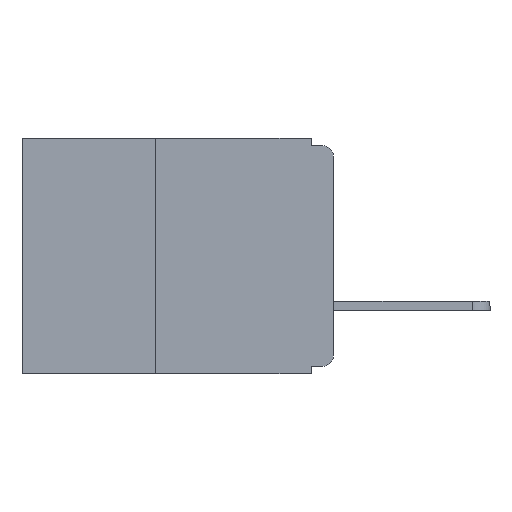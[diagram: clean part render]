
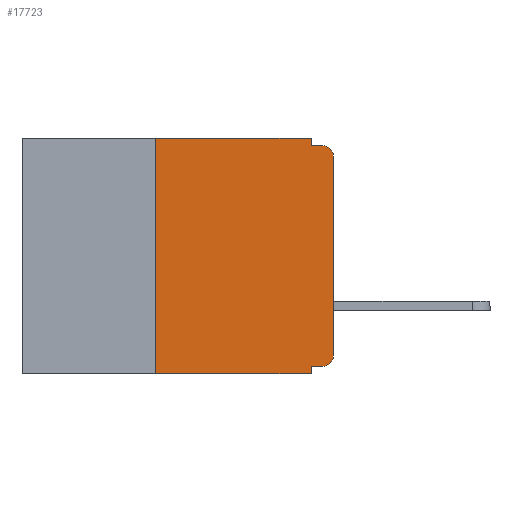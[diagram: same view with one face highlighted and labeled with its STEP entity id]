
A CAD part, left-side view. The second image highlights one B-rep face of the part: STEP entity #17723.
In plain terms, the highlighted planar face has unit normal (-1, 0, 0).
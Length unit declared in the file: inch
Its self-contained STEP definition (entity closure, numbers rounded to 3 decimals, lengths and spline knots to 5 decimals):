
#529 = AXIS2_PLACEMENT_3D ( 'NONE', #19629, #15218, #2746 ) ;
#1301 = EDGE_CURVE ( 'NONE', #6737, #12225, #20094, .T. ) ;
#1304 = AXIS2_PLACEMENT_3D ( 'NONE', #9690, #3925, #2881 ) ;
#1954 = VERTEX_POINT ( 'NONE', #9697 ) ;
#2313 = EDGE_CURVE ( 'NONE', #10436, #1954, #17542, .T. ) ;
#2382 = EDGE_CURVE ( 'NONE', #9512, #3164, #15989, .T. ) ;
#2688 = EDGE_CURVE ( 'NONE', #3176, #16818, #7140, .T. ) ;
#2746 = DIRECTION ( 'NONE',  ( 0., 0., -1. ) ) ;
#2881 = DIRECTION ( 'NONE',  ( 0., 0., -1. ) ) ;
#3124 = VECTOR ( 'NONE', #14455, 39.37008 ) ;
#3146 = LINE ( 'NONE', #15169, #3124 ) ;
#3164 = VERTEX_POINT ( 'NONE', #4464 ) ;
#3176 = VERTEX_POINT ( 'NONE', #18216 ) ;
#3925 = DIRECTION ( 'NONE',  ( -1., 0., 0. ) ) ;
#3968 = EDGE_LOOP ( 'NONE', ( #12111, #12404, #12671, #12971, #13162, #13450, #13623, #13916, #14060, #14146 ) ) ;
#4005 = DIRECTION ( 'NONE',  ( 0., -1., 0. ) ) ;
#4006 = VECTOR ( 'NONE', #19740, 39.37008 ) ;
#4296 = CARTESIAN_POINT ( 'NONE',  ( 0., 0., -0.01 ) ) ;
#4464 = CARTESIAN_POINT ( 'NONE',  ( 0., 0., -0.305 ) ) ;
#4554 = LINE ( 'NONE', #20011, #4006 ) ;
#4828 = CARTESIAN_POINT ( 'NONE',  ( 0., 0., 0. ) ) ;
#5099 = LINE ( 'NONE', #7003, #6762 ) ;
#5101 = DIRECTION ( 'NONE',  ( 0., 0., 1. ) ) ;
#5214 = CARTESIAN_POINT ( 'NONE',  ( 0., 0.031, 0. ) ) ;
#6737 = VERTEX_POINT ( 'NONE', #10512 ) ;
#6762 = VECTOR ( 'NONE', #7384, 39.37008 ) ;
#6795 = VERTEX_POINT ( 'NONE', #8122 ) ;
#7003 = CARTESIAN_POINT ( 'NONE',  ( 0., 0.031, 0. ) ) ;
#7140 = CIRCLE ( 'NONE', #1304, 0.015 ) ;
#7384 = DIRECTION ( 'NONE',  ( 0., 0., -1. ) ) ;
#7558 = DIRECTION ( 'NONE',  ( 0., 0., 1. ) ) ;
#8009 = VERTEX_POINT ( 'NONE', #5214 ) ;
#8122 = CARTESIAN_POINT ( 'NONE',  ( 0., 0.031, -0.01 ) ) ;
#9164 = EDGE_CURVE ( 'NONE', #6795, #16818, #11455, .T. ) ;
#9512 = VERTEX_POINT ( 'NONE', #19906 ) ;
#9690 = CARTESIAN_POINT ( 'NONE',  ( 0., 0.015, -0.025 ) ) ;
#9697 = CARTESIAN_POINT ( 'NONE',  ( 0., 0.25, 0. ) ) ;
#10065 = CARTESIAN_POINT ( 'NONE',  ( 0., 0.031, -0.33 ) ) ;
#10436 = VERTEX_POINT ( 'NONE', #17234 ) ;
#10447 = LINE ( 'NONE', #19452, #10653 ) ;
#10512 = CARTESIAN_POINT ( 'NONE',  ( 0., 0.031, -0.32 ) ) ;
#10653 = VECTOR ( 'NONE', #19446, 39.37008 ) ;
#11354 = VECTOR ( 'NONE', #4005, 39.37008 ) ;
#11455 = LINE ( 'NONE', #4296, #11354 ) ;
#12111 = ORIENTED_EDGE ( 'NONE', *, *, #13014, .T. ) ;
#12225 = VERTEX_POINT ( 'NONE', #10065 ) ;
#12404 = ORIENTED_EDGE ( 'NONE', *, *, #2688, .T. ) ;
#12595 = CARTESIAN_POINT ( 'NONE',  ( 0., 0.25, -0.33 ) ) ;
#12671 = ORIENTED_EDGE ( 'NONE', *, *, #9164, .F. ) ;
#12971 = ORIENTED_EDGE ( 'NONE', *, *, #20355, .F. ) ;
#13014 = EDGE_CURVE ( 'NONE', #3164, #3176, #13865, .T. ) ;
#13162 = ORIENTED_EDGE ( 'NONE', *, *, #18551, .F. ) ;
#13450 = ORIENTED_EDGE ( 'NONE', *, *, #2313, .F. ) ;
#13623 = ORIENTED_EDGE ( 'NONE', *, *, #16165, .T. ) ;
#13865 = LINE ( 'NONE', #4828, #13922 ) ;
#13916 = ORIENTED_EDGE ( 'NONE', *, *, #1301, .F. ) ;
#13922 = VECTOR ( 'NONE', #5101, 39.37008 ) ;
#13992 = DIRECTION ( 'NONE',  ( 0., 0., -1. ) ) ;
#14060 = ORIENTED_EDGE ( 'NONE', *, *, #15263, .F. ) ;
#14146 = ORIENTED_EDGE ( 'NONE', *, *, #2382, .T. ) ;
#14455 = DIRECTION ( 'NONE',  ( 0., 1., 0. ) ) ;
#15169 = CARTESIAN_POINT ( 'NONE',  ( 0., 0., -0.32 ) ) ;
#15218 = DIRECTION ( 'NONE',  ( -1., 0., 0. ) ) ;
#15237 = CARTESIAN_POINT ( 'NONE',  ( 0., 0.015, -0.01 ) ) ;
#15263 = EDGE_CURVE ( 'NONE', #9512, #6737, #3146, .T. ) ;
#15360 = FACE_OUTER_BOUND ( 'NONE', #3968, .T. ) ;
#15989 = CIRCLE ( 'NONE', #529, 0.015 ) ;
#16165 = EDGE_CURVE ( 'NONE', #10436, #12225, #4554, .T. ) ;
#16818 = VERTEX_POINT ( 'NONE', #15237 ) ;
#17093 = VECTOR ( 'NONE', #7558, 39.37008 ) ;
#17234 = CARTESIAN_POINT ( 'NONE',  ( 0., 0.25, -0.33 ) ) ;
#17542 = LINE ( 'NONE', #12595, #17093 ) ;
#17723 = ADVANCED_FACE ( 'NONE', ( #15360 ), #17799, .F. ) ;
#17749 = DIRECTION ( 'NONE',  ( 0., 0., -1. ) ) ;
#17753 = DIRECTION ( 'NONE',  ( 1., 0., 0. ) ) ;
#17799 = PLANE ( 'NONE',  #19719 ) ;
#17823 = CARTESIAN_POINT ( 'NONE',  ( 0., 0.031, -0.33 ) ) ;
#18216 = CARTESIAN_POINT ( 'NONE',  ( 0., 0., -0.025 ) ) ;
#18328 = CARTESIAN_POINT ( 'NONE',  ( 0., 0.437, 0. ) ) ;
#18338 = VECTOR ( 'NONE', #13992, 39.37008 ) ;
#18551 = EDGE_CURVE ( 'NONE', #1954, #8009, #10447, .T. ) ;
#19446 = DIRECTION ( 'NONE',  ( 0., -1., 0. ) ) ;
#19452 = CARTESIAN_POINT ( 'NONE',  ( 0., 0.437, 0. ) ) ;
#19629 = CARTESIAN_POINT ( 'NONE',  ( 0., 0.015, -0.305 ) ) ;
#19719 = AXIS2_PLACEMENT_3D ( 'NONE', #18328, #17753, #17749 ) ;
#19740 = DIRECTION ( 'NONE',  ( 0., -1., 0. ) ) ;
#19906 = CARTESIAN_POINT ( 'NONE',  ( 0., 0.015, -0.32 ) ) ;
#20011 = CARTESIAN_POINT ( 'NONE',  ( 0., 0.437, -0.33 ) ) ;
#20094 = LINE ( 'NONE', #17823, #18338 ) ;
#20355 = EDGE_CURVE ( 'NONE', #8009, #6795, #5099, .T. ) ;
